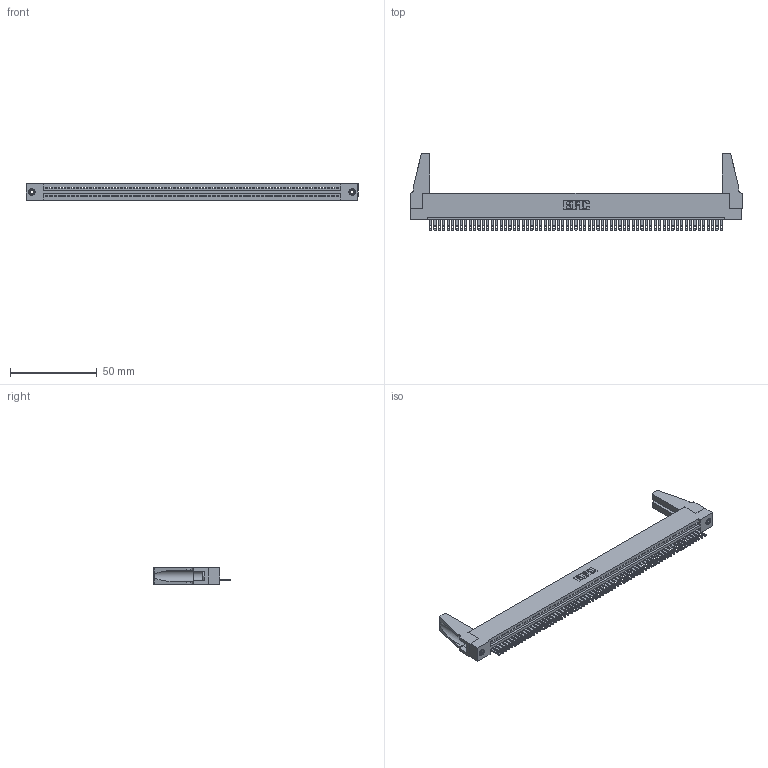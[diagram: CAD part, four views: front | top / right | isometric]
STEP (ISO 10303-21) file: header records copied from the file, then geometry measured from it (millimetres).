
FILE_DESCRIPTION (( 'STEP AP203' ), '1' );
FILE_NAME ('345-067-500-188.STEP', '2019-10-11T23:32:00', ( '' ), ( '' ), 'SwSTEP 2.0', 'SolidWorks 2016', '' );
FILE_SCHEMA (( 'CONFIG_CONTROL_DESIGN' ));
Length unit declared in the file: inch
Products named in the file (5): 345-067-500-188; 345-220-078_345-220-088; 345 Part_Flush Mounting Lugs - 0.156 Dia-TH; 345-292-001_345-293-100; 345-250-001_345-250-001-102
Assembly tree (72 placements, depth 2):
  345-067-500-188
    345 Part_Flush Mounting Lugs - 0.156 Dia-TH
    345-292-001_345-293-100  x67
    345-250-001_345-250-001-102  x2
    345-220-078_345-220-088  x2
Bounding box: 191.41 x 44.37 x 9.4 mm (x, y, z)
Volume: 21679.5 mm3; surface area: 28107.3 mm2
Topology: 72 solids, 72 shells, 3868 faces, 11911 edges, 7930 vertices
Faces by surface type: plane 2430, cylinder 1422, cone 12, torus 4
Entity records: 49138 total; most frequent: CARTESIAN_POINT 8499, ORIENTED_EDGE 8460, DIRECTION 7396, EDGE_CURVE 4230, LINE 3784, VECTOR 3784, VERTEX_POINT 2814, AXIS2_PLACEMENT_3D 1806
